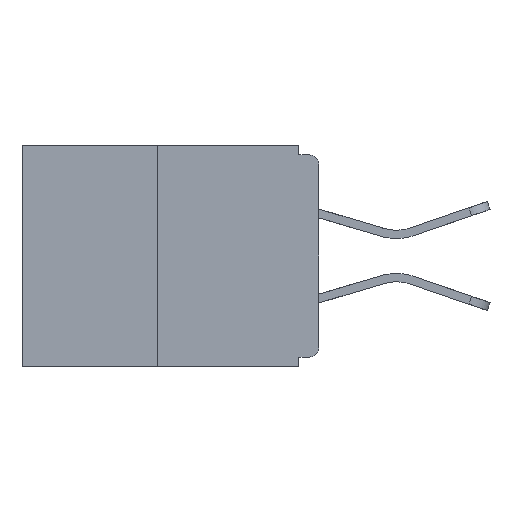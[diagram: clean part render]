
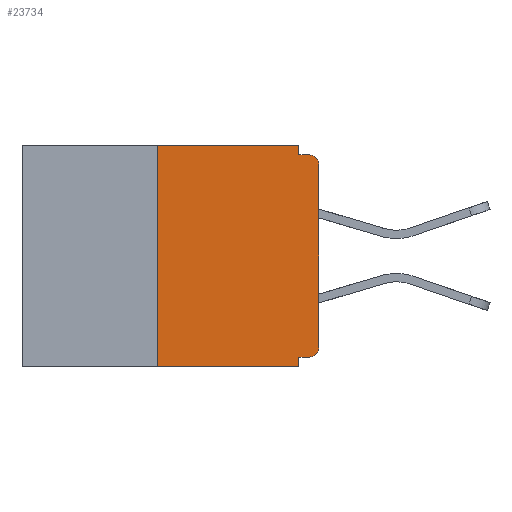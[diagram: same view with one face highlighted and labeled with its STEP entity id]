
A CAD part, left-side view. The second image highlights one B-rep face of the part: STEP entity #23734.
In plain terms, the highlighted planar face has unit normal (-1, 0, 0).
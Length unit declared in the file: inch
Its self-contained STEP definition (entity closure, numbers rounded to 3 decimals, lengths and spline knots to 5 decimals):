
#3 = CARTESIAN_POINT ( 'NONE',  ( 0., 0.031, 0. ) ) ;
#432 = VERTEX_POINT ( 'NONE', #14884 ) ;
#467 = EDGE_LOOP ( 'NONE', ( #21864, #13056, #14951, #16467, #702, #5961, #17127, #27517, #17690, #26626 ) ) ;
#702 = ORIENTED_EDGE ( 'NONE', *, *, #27104, .F. ) ;
#1574 = CARTESIAN_POINT ( 'NONE',  ( 0., 0.25, 0. ) ) ;
#3121 = EDGE_CURVE ( 'NONE', #7351, #19567, #20820, .T. ) ;
#3127 = CARTESIAN_POINT ( 'NONE',  ( 0., 0.015, -0.03 ) ) ;
#3588 = LINE ( 'NONE', #28215, #8007 ) ;
#3756 = CARTESIAN_POINT ( 'NONE',  ( 0., 0., -0.03 ) ) ;
#4532 = EDGE_CURVE ( 'NONE', #28134, #24813, #17313, .T. ) ;
#5554 = DIRECTION ( 'NONE',  ( 0., -1., 0. ) ) ;
#5731 = DIRECTION ( 'NONE',  ( 0., 0., 1. ) ) ;
#5867 = CIRCLE ( 'NONE', #18125, 0.015 ) ;
#5961 = ORIENTED_EDGE ( 'NONE', *, *, #7552, .T. ) ;
#6157 = CARTESIAN_POINT ( 'NONE',  ( 0., 0.031, 0. ) ) ;
#6267 = AXIS2_PLACEMENT_3D ( 'NONE', #25037, #10027, #24852 ) ;
#6536 = LINE ( 'NONE', #1574, #18134 ) ;
#6977 = DIRECTION ( 'NONE',  ( -1., 0., 0. ) ) ;
#7351 = VERTEX_POINT ( 'NONE', #20945 ) ;
#7417 = VERTEX_POINT ( 'NONE', #13097 ) ;
#7552 = EDGE_CURVE ( 'NONE', #22825, #7351, #5867, .T. ) ;
#8007 = VECTOR ( 'NONE', #21544, 39.37008 ) ;
#8074 = CARTESIAN_POINT ( 'NONE',  ( 0., 0.015, -0.015 ) ) ;
#8234 = DIRECTION ( 'NONE',  ( 0., 0., 1. ) ) ;
#8658 = CARTESIAN_POINT ( 'NONE',  ( 0., 0.25, 0. ) ) ;
#8751 = VECTOR ( 'NONE', #20644, 39.37008 ) ;
#10027 = DIRECTION ( 'NONE',  ( 1., 0., 0. ) ) ;
#10502 = EDGE_CURVE ( 'NONE', #19567, #24810, #10689, .T. ) ;
#10689 = CIRCLE ( 'NONE', #26754, 0.015 ) ;
#11306 = DIRECTION ( 'NONE',  ( 0., 0., -1. ) ) ;
#11423 = CARTESIAN_POINT ( 'NONE',  ( 0., 0., -0.328 ) ) ;
#11508 = VECTOR ( 'NONE', #14907, 39.37008 ) ;
#12053 = FACE_OUTER_BOUND ( 'NONE', #467, .T. ) ;
#12553 = CARTESIAN_POINT ( 'NONE',  ( 0., 0.46, -0.343 ) ) ;
#12740 = DIRECTION ( 'NONE',  ( 0., -1., 0. ) ) ;
#13056 = ORIENTED_EDGE ( 'NONE', *, *, #17225, .F. ) ;
#13097 = CARTESIAN_POINT ( 'NONE',  ( 0., 0.031, -0.343 ) ) ;
#13910 = EDGE_CURVE ( 'NONE', #432, #7417, #19691, .T. ) ;
#14719 = CARTESIAN_POINT ( 'NONE',  ( 0., 0., -0.015 ) ) ;
#14884 = CARTESIAN_POINT ( 'NONE',  ( 0., 0.031, -0.328 ) ) ;
#14907 = DIRECTION ( 'NONE',  ( 0., 0., -1. ) ) ;
#14951 = ORIENTED_EDGE ( 'NONE', *, *, #23184, .T. ) ;
#15359 = VECTOR ( 'NONE', #5731, 39.37008 ) ;
#15390 = CARTESIAN_POINT ( 'NONE',  ( 0., 0.015, -0.313 ) ) ;
#15824 = DIRECTION ( 'NONE',  ( 0., 0., -1. ) ) ;
#16467 = ORIENTED_EDGE ( 'NONE', *, *, #13910, .F. ) ;
#17127 = ORIENTED_EDGE ( 'NONE', *, *, #3121, .T. ) ;
#17225 = EDGE_CURVE ( 'NONE', #22094, #18667, #6536, .T. ) ;
#17313 = LINE ( 'NONE', #3, #11508 ) ;
#17690 = ORIENTED_EDGE ( 'NONE', *, *, #27188, .F. ) ;
#18125 = AXIS2_PLACEMENT_3D ( 'NONE', #15390, #6977, #11306 ) ;
#18134 = VECTOR ( 'NONE', #8234, 39.37008 ) ;
#18348 = LINE ( 'NONE', #11423, #8751 ) ;
#18413 = DIRECTION ( 'NONE',  ( -1., 0., 0. ) ) ;
#18667 = VERTEX_POINT ( 'NONE', #8658 ) ;
#18992 = CARTESIAN_POINT ( 'NONE',  ( 0., 0.031, -0.015 ) ) ;
#19467 = DIRECTION ( 'NONE',  ( 0., 0., -1. ) ) ;
#19567 = VERTEX_POINT ( 'NONE', #3756 ) ;
#19691 = LINE ( 'NONE', #19795, #20374 ) ;
#19795 = CARTESIAN_POINT ( 'NONE',  ( 0., 0.031, -0.343 ) ) ;
#20205 = CARTESIAN_POINT ( 'NONE',  ( 0., 0.25, -0.343 ) ) ;
#20282 = VECTOR ( 'NONE', #12740, 39.37008 ) ;
#20374 = VECTOR ( 'NONE', #19467, 39.37008 ) ;
#20644 = DIRECTION ( 'NONE',  ( 0., 1., 0. ) ) ;
#20705 = LINE ( 'NONE', #14719, #22408 ) ;
#20732 = CARTESIAN_POINT ( 'NONE',  ( 0., 0., 0. ) ) ;
#20820 = LINE ( 'NONE', #20732, #15359 ) ;
#20945 = CARTESIAN_POINT ( 'NONE',  ( 0., 0., -0.313 ) ) ;
#21544 = DIRECTION ( 'NONE',  ( 0., -1., 0. ) ) ;
#21864 = ORIENTED_EDGE ( 'NONE', *, *, #27780, .F. ) ;
#22094 = VERTEX_POINT ( 'NONE', #20205 ) ;
#22408 = VECTOR ( 'NONE', #5554, 39.37008 ) ;
#22770 = CARTESIAN_POINT ( 'NONE',  ( 0., 0.015, -0.328 ) ) ;
#22825 = VERTEX_POINT ( 'NONE', #22770 ) ;
#23184 = EDGE_CURVE ( 'NONE', #22094, #7417, #26064, .T. ) ;
#23734 = ADVANCED_FACE ( 'NONE', ( #12053 ), #24942, .F. ) ;
#24810 = VERTEX_POINT ( 'NONE', #8074 ) ;
#24813 = VERTEX_POINT ( 'NONE', #18992 ) ;
#24852 = DIRECTION ( 'NONE',  ( 0., 0., -1. ) ) ;
#24942 = PLANE ( 'NONE',  #6267 ) ;
#25037 = CARTESIAN_POINT ( 'NONE',  ( 0., 0.46, 0. ) ) ;
#26064 = LINE ( 'NONE', #12553, #20282 ) ;
#26626 = ORIENTED_EDGE ( 'NONE', *, *, #4532, .F. ) ;
#26754 = AXIS2_PLACEMENT_3D ( 'NONE', #3127, #18413, #15824 ) ;
#27104 = EDGE_CURVE ( 'NONE', #22825, #432, #18348, .T. ) ;
#27188 = EDGE_CURVE ( 'NONE', #24813, #24810, #20705, .T. ) ;
#27517 = ORIENTED_EDGE ( 'NONE', *, *, #10502, .T. ) ;
#27780 = EDGE_CURVE ( 'NONE', #18667, #28134, #3588, .T. ) ;
#28134 = VERTEX_POINT ( 'NONE', #6157 ) ;
#28215 = CARTESIAN_POINT ( 'NONE',  ( 0., 0.46, 0. ) ) ;
